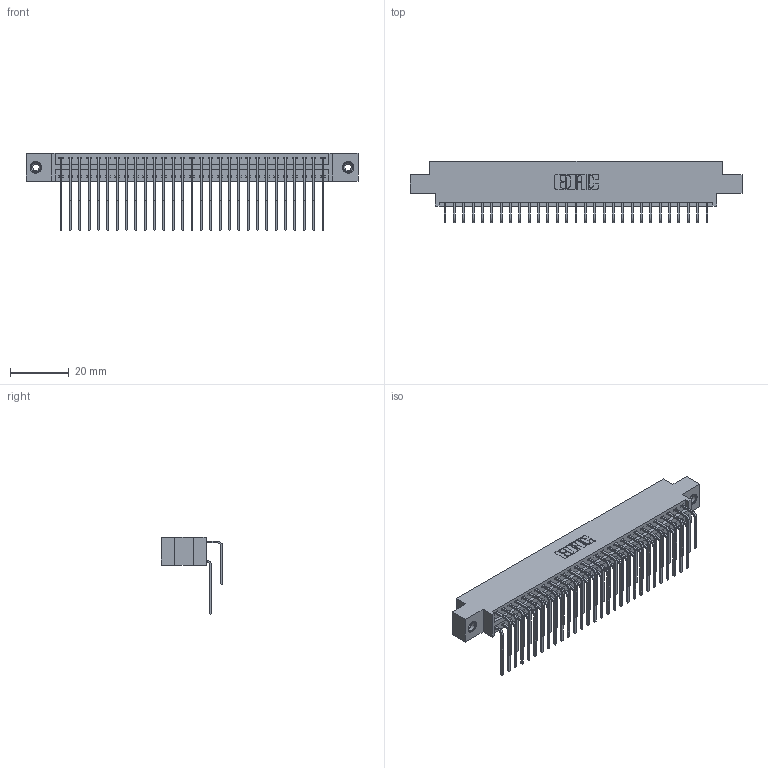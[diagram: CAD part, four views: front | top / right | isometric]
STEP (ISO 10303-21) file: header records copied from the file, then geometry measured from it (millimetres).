
FILE_DESCRIPTION (( 'STEP AP203' ), '1' );
FILE_NAME ('396-058-559-808.STEP', '2019-11-03T09:40:23', ( '' ), ( '' ), 'SwSTEP 2.0', 'SolidWorks 2016', '' );
FILE_SCHEMA (( 'CONFIG_CONTROL_DESIGN' ));
Length unit declared in the file: inch
Products named in the file (5): 396-058-559-808; 345-250-001_345-250-003-102; 346 Part_0.170 Offset - 0.156 Dia-TI; 345-292-001_559 Tail - 2; 345-292-001_558 559 Tail - 1
Assembly tree (61 placements, depth 2):
  396-058-559-808
    346 Part_0.170 Offset - 0.156 Dia-TI
    345-292-001_558 559 Tail - 1  x29
    345-292-001_559 Tail - 2  x29
    345-250-001_345-250-003-102  x2
Bounding box: 112.65 x 20.89 x 26.16 mm (x, y, z)
Volume: 11057.2 mm3; surface area: 16799.3 mm2
Topology: 61 solids, 61 shells, 3318 faces, 9815 edges, 6458 vertices
Faces by surface type: plane 2258, cylinder 1044, cone 12, torus 4
Entity records: 23778 total; most frequent: CARTESIAN_POINT 3974, ORIENTED_EDGE 3850, DIRECTION 3551, EDGE_CURVE 1925, VECTOR 1617, LINE 1617, VERTEX_POINT 1276, AXIS2_PLACEMENT_3D 967
